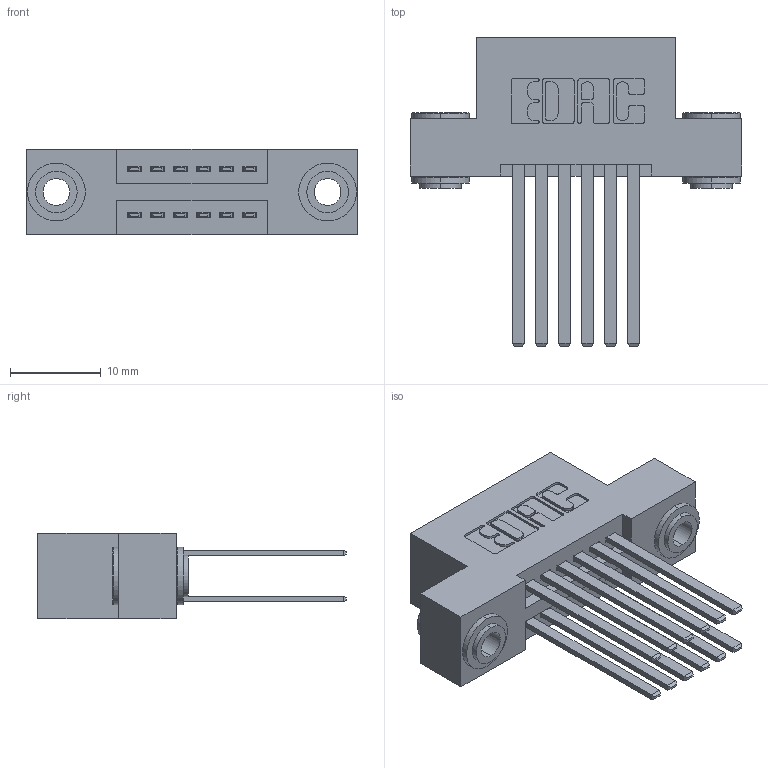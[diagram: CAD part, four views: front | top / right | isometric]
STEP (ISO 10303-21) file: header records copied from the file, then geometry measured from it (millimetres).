
FILE_DESCRIPTION (( 'STEP AP203' ), '1' );
FILE_NAME ('345-012-544-203.STEP', '2019-10-26T16:26:15', ( '' ), ( '' ), 'SwSTEP 2.0', 'SolidWorks 2016', '' );
FILE_SCHEMA (( 'CONFIG_CONTROL_DESIGN' ));
Length unit declared in the file: inch
Products named in the file (4): 345-250-002_345-250-002-102; 345 Part_Flush Mounting Lugs - 0.156 Dia-TH; 345-012-544-203; 345-292-001_345-293-144
Assembly tree (15 placements, depth 2):
  345-012-544-203
    345 Part_Flush Mounting Lugs - 0.156 Dia-TH
    345-292-001_345-293-144  x12
    345-250-002_345-250-002-102  x2
Bounding box: 36.45 x 33.96 x 9.4 mm (x, y, z)
Volume: 3394.1 mm3; surface area: 5017.8 mm2
Topology: 15 solids, 15 shells, 692 faces, 1989 edges, 1306 vertices
Faces by surface type: plane 438, cylinder 246, cone 8
Entity records: 10020 total; most frequent: CARTESIAN_POINT 1687, ORIENTED_EDGE 1614, DIRECTION 1561, EDGE_CURVE 807, VECTOR 631, LINE 631, VERTEX_POINT 534, AXIS2_PLACEMENT_3D 465
